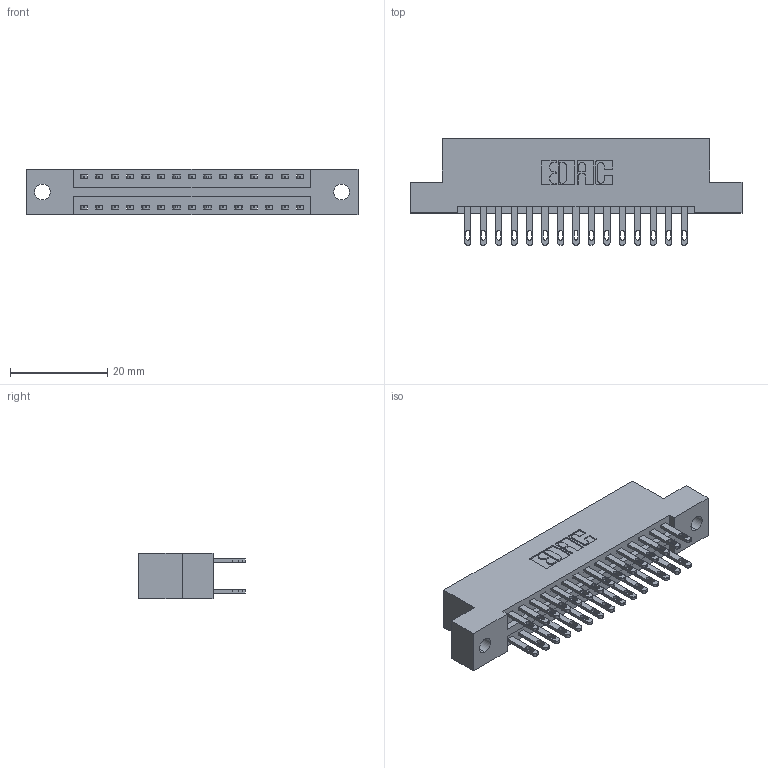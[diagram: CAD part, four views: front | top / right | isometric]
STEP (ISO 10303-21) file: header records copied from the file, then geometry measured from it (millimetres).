
FILE_DESCRIPTION (( 'STEP AP203' ), '1' );
FILE_NAME ('896-030-500-202.STEP', '2021-07-27T18:46:20', ( '' ), ( '' ), 'SwSTEP 2.0', 'SolidWorks 2020', '' );
FILE_SCHEMA (( 'CONFIG_CONTROL_DESIGN' ));
Length unit declared in the file: inch
Products named in the file (3): 846 Part_Flush Mounting Lugs - 0.128 Dia; 345-292-001_345-293-100; 896-030-500-202
Assembly tree (31 placements, depth 2):
  896-030-500-202
    846 Part_Flush Mounting Lugs - 0.128 Dia
    345-292-001_345-293-100  x30
Bounding box: 68.2 x 21.84 x 9.4 mm (x, y, z)
Volume: 6495.5 mm3; surface area: 8548.9 mm2
Topology: 31 solids, 31 shells, 1562 faces, 4739 edges, 3158 vertices
Faces by surface type: plane 946, cylinder 616
Entity records: 13357 total; most frequent: CARTESIAN_POINT 2236, ORIENTED_EDGE 2170, DIRECTION 2025, EDGE_CURVE 1085, LINE 889, VECTOR 889, VERTEX_POINT 722, AXIS2_PLACEMENT_3D 568
